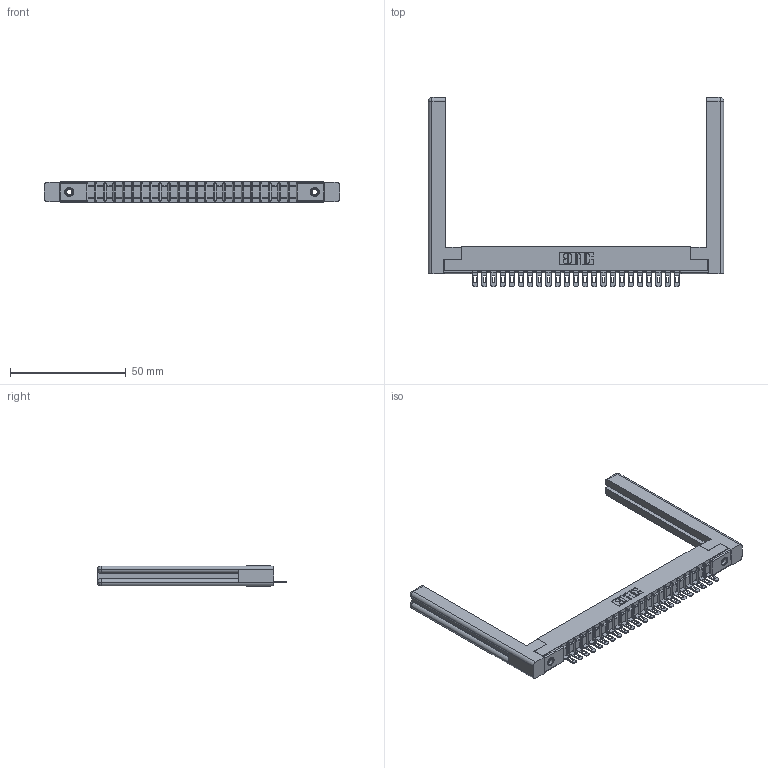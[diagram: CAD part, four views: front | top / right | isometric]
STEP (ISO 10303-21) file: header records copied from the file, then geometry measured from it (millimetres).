
FILE_DESCRIPTION (( 'STEP AP203' ), '1' );
FILE_NAME ('357-023-501-158.STEP', '2019-09-16T23:32:57', ( '' ), ( '' ), 'SwSTEP 2.0', 'SolidWorks 2016', '' );
FILE_SCHEMA (( 'CONFIG_CONTROL_DESIGN' ));
Length unit declared in the file: inch
Products named in the file (5): 357-023-501-158; 307-290-002_501; 307 Part_.156 Dia Mounting Holes; 345-250-001_345-250-001-102; 307-220-058
Assembly tree (28 placements, depth 2):
  357-023-501-158
    307 Part_.156 Dia Mounting Holes
    307-290-002_501  x23
    307-220-058  x2
    345-250-001_345-250-001-102  x2
Bounding box: 127.76 x 81.74 x 8.71 mm (x, y, z)
Volume: 16133.5 mm3; surface area: 20613.3 mm2
Topology: 28 solids, 28 shells, 2032 faces, 6151 edges, 4022 vertices
Faces by surface type: plane 1166, cylinder 794, sphere 48, torus 12, cone 12
Entity records: 25487 total; most frequent: CARTESIAN_POINT 4303, ORIENTED_EDGE 4232, DIRECTION 4154, EDGE_CURVE 2116, VECTOR 1604, LINE 1604, VERTEX_POINT 1370, AXIS2_PLACEMENT_3D 1275
